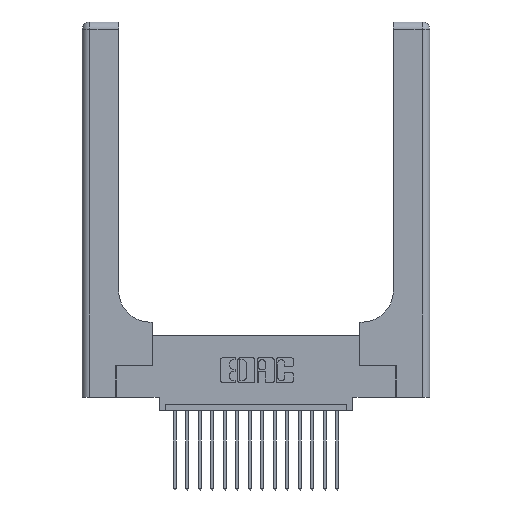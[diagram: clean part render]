
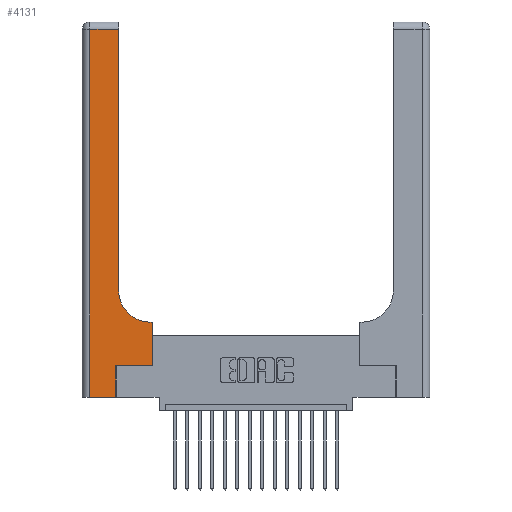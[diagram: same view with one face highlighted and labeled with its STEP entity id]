
A CAD part, top view. The second image highlights one B-rep face of the part: STEP entity #4131.
In plain terms, the highlighted planar face has unit normal (0, 0, 1).
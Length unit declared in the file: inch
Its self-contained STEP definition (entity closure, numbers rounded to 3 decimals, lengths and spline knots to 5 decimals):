
#155 = VERTEX_POINT ( 'NONE', #1671 ) ;
#182 = EDGE_LOOP ( 'NONE', ( #9516, #10753, #13404, #13181, #6261, #10707, #15753, #3004, #10122 ) ) ;
#315 = EDGE_CURVE ( 'NONE', #14592, #6688, #17209, .T. ) ;
#751 = AXIS2_PLACEMENT_3D ( 'NONE', #2013, #8183, #12482 ) ;
#1671 = CARTESIAN_POINT ( 'NONE',  ( 0.2915, 2.94, 0.37 ) ) ;
#1702 = DIRECTION ( 'NONE',  ( -1., 0., 0. ) ) ;
#2013 = CARTESIAN_POINT ( 'NONE',  ( 0.5415, 0.85, 0.37 ) ) ;
#2289 = CARTESIAN_POINT ( 'NONE',  ( 0.269, 0., 0.37 ) ) ;
#2399 = VERTEX_POINT ( 'NONE', #4202 ) ;
#2412 = VERTEX_POINT ( 'NONE', #2711 ) ;
#2711 = CARTESIAN_POINT ( 'NONE',  ( 0.269, 0.25, 0.37 ) ) ;
#2922 = CARTESIAN_POINT ( 'NONE',  ( 0.5415, 0.6, 0.37 ) ) ;
#3004 = ORIENTED_EDGE ( 'NONE', *, *, #11422, .T. ) ;
#3303 = CARTESIAN_POINT ( 'NONE',  ( 0.269, 0.25, 0.37 ) ) ;
#3522 = LINE ( 'NONE', #4585, #17332 ) ;
#3856 = LINE ( 'NONE', #18570, #10530 ) ;
#4131 = ADVANCED_FACE ( 'NONE', ( #18803 ), #15060, .F. ) ;
#4202 = CARTESIAN_POINT ( 'NONE',  ( 0.06, 2.94, 0.37 ) ) ;
#4265 = VERTEX_POINT ( 'NONE', #2289 ) ;
#4585 = CARTESIAN_POINT ( 'NONE',  ( 0.5585, 0.25, 0.37 ) ) ;
#5259 = LINE ( 'NONE', #13590, #11254 ) ;
#5383 = VECTOR ( 'NONE', #1702, 39.37008 ) ;
#5389 = VECTOR ( 'NONE', #17803, 39.37008 ) ;
#5601 = EDGE_CURVE ( 'NONE', #14892, #4265, #3856, .T. ) ;
#5686 = DIRECTION ( 'NONE',  ( 0., 1., 0. ) ) ;
#5892 = DIRECTION ( 'NONE',  ( -1., 0., 0. ) ) ;
#6261 = ORIENTED_EDGE ( 'NONE', *, *, #8803, .T. ) ;
#6360 = LINE ( 'NONE', #7803, #5383 ) ;
#6688 = VERTEX_POINT ( 'NONE', #17631 ) ;
#6997 = LINE ( 'NONE', #3303, #10091 ) ;
#7214 = DIRECTION ( 'NONE',  ( 0., -1., 0. ) ) ;
#7579 = VECTOR ( 'NONE', #5686, 39.37008 ) ;
#7803 = CARTESIAN_POINT ( 'NONE',  ( 0.2915, 0.6, 0.37 ) ) ;
#7854 = EDGE_CURVE ( 'NONE', #2399, #14892, #9490, .T. ) ;
#8183 = DIRECTION ( 'NONE',  ( 0., 0., -1. ) ) ;
#8636 = EDGE_CURVE ( 'NONE', #16279, #19314, #3522, .T. ) ;
#8652 = CARTESIAN_POINT ( 'NONE',  ( 0.269, 0., 0.37 ) ) ;
#8766 = EDGE_CURVE ( 'NONE', #6688, #155, #18970, .T. ) ;
#8789 = DIRECTION ( 'NONE',  ( 0., 0., -1. ) ) ;
#8803 = EDGE_CURVE ( 'NONE', #4265, #2412, #11128, .T. ) ;
#8878 = CARTESIAN_POINT ( 'NONE',  ( 0.5585, 0.6, 0.37 ) ) ;
#9490 = LINE ( 'NONE', #10070, #12607 ) ;
#9516 = ORIENTED_EDGE ( 'NONE', *, *, #8766, .T. ) ;
#10070 = CARTESIAN_POINT ( 'NONE',  ( 0.06, 3., 0.37 ) ) ;
#10091 = VECTOR ( 'NONE', #18761, 39.37008 ) ;
#10122 = ORIENTED_EDGE ( 'NONE', *, *, #315, .T. ) ;
#10530 = VECTOR ( 'NONE', #11209, 39.37008 ) ;
#10707 = ORIENTED_EDGE ( 'NONE', *, *, #18925, .T. ) ;
#10753 = ORIENTED_EDGE ( 'NONE', *, *, #15234, .T. ) ;
#11128 = LINE ( 'NONE', #8652, #5389 ) ;
#11209 = DIRECTION ( 'NONE',  ( 1., 0., 0. ) ) ;
#11254 = VECTOR ( 'NONE', #18125, 39.37008 ) ;
#11422 = EDGE_CURVE ( 'NONE', #19314, #14592, #6360, .T. ) ;
#12482 = DIRECTION ( 'NONE',  ( 1., 0., 0. ) ) ;
#12607 = VECTOR ( 'NONE', #7214, 39.37008 ) ;
#13181 = ORIENTED_EDGE ( 'NONE', *, *, #5601, .T. ) ;
#13265 = CARTESIAN_POINT ( 'NONE',  ( 0.2915, 3., 0.37 ) ) ;
#13404 = ORIENTED_EDGE ( 'NONE', *, *, #7854, .T. ) ;
#13590 = CARTESIAN_POINT ( 'NONE',  ( 0., 2.94, 0.37 ) ) ;
#13880 = DIRECTION ( 'NONE',  ( 0., 1., 0. ) ) ;
#14592 = VERTEX_POINT ( 'NONE', #2922 ) ;
#14687 = CARTESIAN_POINT ( 'NONE',  ( 0.06, 0., 0.37 ) ) ;
#14892 = VERTEX_POINT ( 'NONE', #14687 ) ;
#15060 = PLANE ( 'NONE',  #16312 ) ;
#15234 = EDGE_CURVE ( 'NONE', #155, #2399, #5259, .T. ) ;
#15330 = CARTESIAN_POINT ( 'NONE',  ( 0.5585, 0.25, 0.37 ) ) ;
#15753 = ORIENTED_EDGE ( 'NONE', *, *, #8636, .T. ) ;
#16279 = VERTEX_POINT ( 'NONE', #15330 ) ;
#16312 = AXIS2_PLACEMENT_3D ( 'NONE', #17893, #8789, #5892 ) ;
#17209 = CIRCLE ( 'NONE', #751, 0.25 ) ;
#17332 = VECTOR ( 'NONE', #13880, 39.37008 ) ;
#17631 = CARTESIAN_POINT ( 'NONE',  ( 0.2915, 0.85, 0.37 ) ) ;
#17803 = DIRECTION ( 'NONE',  ( 0., 1., 0. ) ) ;
#17893 = CARTESIAN_POINT ( 'NONE',  ( 0., 3., 0.37 ) ) ;
#18125 = DIRECTION ( 'NONE',  ( -1., 0., 0. ) ) ;
#18570 = CARTESIAN_POINT ( 'NONE',  ( 0., 0., 0.37 ) ) ;
#18761 = DIRECTION ( 'NONE',  ( 1., 0., 0. ) ) ;
#18803 = FACE_OUTER_BOUND ( 'NONE', #182, .T. ) ;
#18925 = EDGE_CURVE ( 'NONE', #2412, #16279, #6997, .T. ) ;
#18970 = LINE ( 'NONE', #13265, #7579 ) ;
#19314 = VERTEX_POINT ( 'NONE', #8878 ) ;
